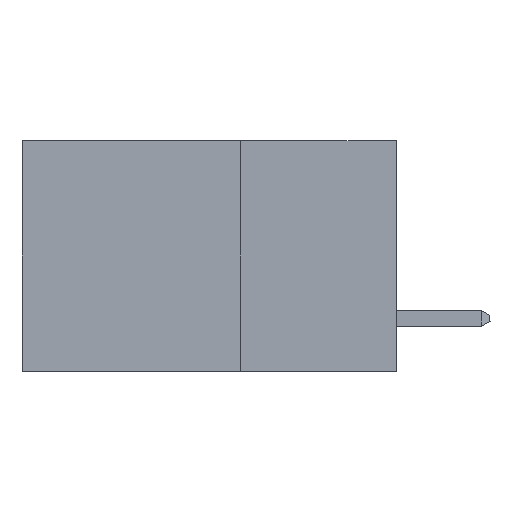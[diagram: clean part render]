
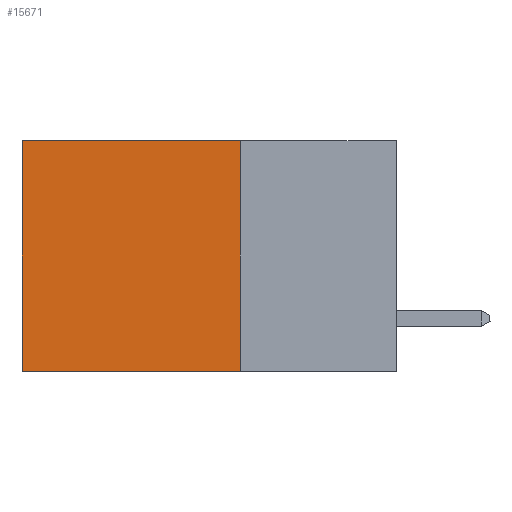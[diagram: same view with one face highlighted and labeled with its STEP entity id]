
A CAD part, left-side view. The second image highlights one B-rep face of the part: STEP entity #15671.
In plain terms, the highlighted planar face has unit normal (-1, 0, 0).
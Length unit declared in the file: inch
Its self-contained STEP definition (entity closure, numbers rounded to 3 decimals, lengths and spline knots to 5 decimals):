
#980 = DIRECTION ( 'NONE',  ( 0., 0., -1. ) ) ;
#1121 = EDGE_CURVE ( 'NONE', #1361, #6122, #21261, .T. ) ;
#1361 = VERTEX_POINT ( 'NONE', #5969 ) ;
#2505 = VECTOR ( 'NONE', #7453, 39.37008 ) ;
#3391 = LINE ( 'NONE', #22226, #3691 ) ;
#3691 = VECTOR ( 'NONE', #16262, 39.37008 ) ;
#3970 = DIRECTION ( 'NONE',  ( 1., 0., 0. ) ) ;
#4286 = LINE ( 'NONE', #21248, #15110 ) ;
#5837 = PLANE ( 'NONE',  #15385 ) ;
#5969 = CARTESIAN_POINT ( 'NONE',  ( 0.298, 0.25, -0.37 ) ) ;
#6098 = VERTEX_POINT ( 'NONE', #26295 ) ;
#6122 = VERTEX_POINT ( 'NONE', #14585 ) ;
#6190 = CARTESIAN_POINT ( 'NONE',  ( 0.298, 0.25, 0. ) ) ;
#6214 = ORIENTED_EDGE ( 'NONE', *, *, #1121, .F. ) ;
#7338 = EDGE_LOOP ( 'NONE', ( #25710, #6214, #15413, #19124 ) ) ;
#7453 = DIRECTION ( 'NONE',  ( 0., 1., 0. ) ) ;
#7735 = CARTESIAN_POINT ( 'NONE',  ( 0.298, 0.25, -0.37 ) ) ;
#7744 = FACE_OUTER_BOUND ( 'NONE', #7338, .T. ) ;
#8163 = DIRECTION ( 'NONE',  ( 0., 0., -1. ) ) ;
#8775 = EDGE_CURVE ( 'NONE', #6098, #6122, #4286, .T. ) ;
#10796 = VECTOR ( 'NONE', #15727, 39.37008 ) ;
#12300 = VERTEX_POINT ( 'NONE', #15115 ) ;
#12333 = EDGE_CURVE ( 'NONE', #12300, #6098, #22216, .T. ) ;
#12908 = CARTESIAN_POINT ( 'NONE',  ( 0.298, 0.25, 0. ) ) ;
#14585 = CARTESIAN_POINT ( 'NONE',  ( 0.298, 0.6, -0.37 ) ) ;
#15110 = VECTOR ( 'NONE', #980, 39.37008 ) ;
#15115 = CARTESIAN_POINT ( 'NONE',  ( 0.298, 0.25, 0. ) ) ;
#15385 = AXIS2_PLACEMENT_3D ( 'NONE', #6190, #3970, #8163 ) ;
#15413 = ORIENTED_EDGE ( 'NONE', *, *, #24634, .F. ) ;
#15671 = ADVANCED_FACE ( 'NONE', ( #7744 ), #5837, .F. ) ;
#15727 = DIRECTION ( 'NONE',  ( 0., 1., 0. ) ) ;
#16262 = DIRECTION ( 'NONE',  ( 0., 0., -1. ) ) ;
#19124 = ORIENTED_EDGE ( 'NONE', *, *, #12333, .T. ) ;
#21248 = CARTESIAN_POINT ( 'NONE',  ( 0.298, 0.6, 0. ) ) ;
#21261 = LINE ( 'NONE', #7735, #10796 ) ;
#22216 = LINE ( 'NONE', #12908, #2505 ) ;
#22226 = CARTESIAN_POINT ( 'NONE',  ( 0.298, 0.25, 0. ) ) ;
#24634 = EDGE_CURVE ( 'NONE', #12300, #1361, #3391, .T. ) ;
#25710 = ORIENTED_EDGE ( 'NONE', *, *, #8775, .T. ) ;
#26295 = CARTESIAN_POINT ( 'NONE',  ( 0.298, 0.6, 0. ) ) ;
